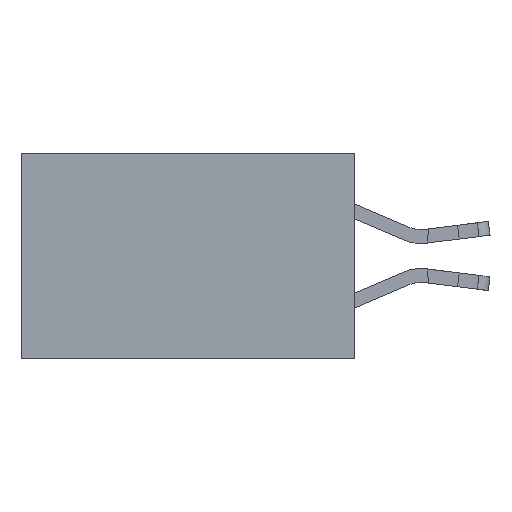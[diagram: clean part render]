
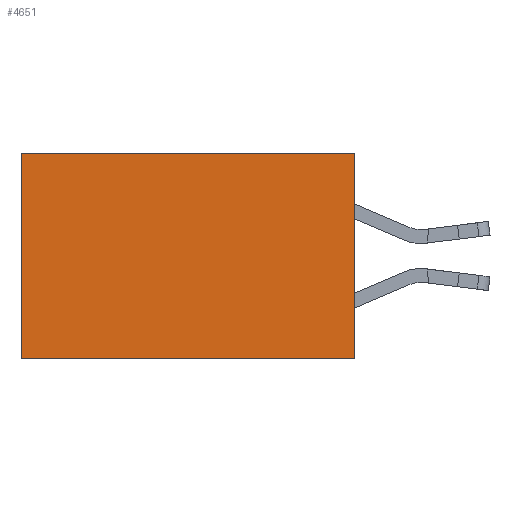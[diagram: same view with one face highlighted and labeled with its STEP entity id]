
A CAD part, left-side view. The second image highlights one B-rep face of the part: STEP entity #4651.
In plain terms, the highlighted planar face has unit normal (-1, 0, 0).
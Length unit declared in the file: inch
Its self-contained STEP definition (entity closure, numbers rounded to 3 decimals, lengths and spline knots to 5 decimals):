
#107 = CARTESIAN_POINT ( 'NONE',  ( 0.2615, 0.6, -0.37 ) ) ;
#495 = AXIS2_PLACEMENT_3D ( 'NONE', #16138, #16230, #9547 ) ;
#977 = VECTOR ( 'NONE', #4825, 39.37008 ) ;
#1746 = DIRECTION ( 'NONE',  ( 0., 1., 0. ) ) ;
#3487 = EDGE_CURVE ( 'NONE', #14373, #7581, #16564, .T. ) ;
#3870 = VECTOR ( 'NONE', #1746, 39.37008 ) ;
#4035 = EDGE_LOOP ( 'NONE', ( #16131, #14658, #6083, #10018 ) ) ;
#4062 = DIRECTION ( 'NONE',  ( 0., 0., -1. ) ) ;
#4365 = VERTEX_POINT ( 'NONE', #107 ) ;
#4651 = ADVANCED_FACE ( 'NONE', ( #12089 ), #7894, .F. ) ;
#4653 = CARTESIAN_POINT ( 'NONE',  ( 0.2615, 0.6, 0. ) ) ;
#4825 = DIRECTION ( 'NONE',  ( 0., 1., 0. ) ) ;
#5568 = CARTESIAN_POINT ( 'NONE',  ( 0.2615, 0., -0.37 ) ) ;
#6083 = ORIENTED_EDGE ( 'NONE', *, *, #12472, .F. ) ;
#6789 = LINE ( 'NONE', #5568, #12208 ) ;
#7273 = CARTESIAN_POINT ( 'NONE',  ( 0.2615, 0., -0.37 ) ) ;
#7565 = DIRECTION ( 'NONE',  ( 0., 0., -1. ) ) ;
#7581 = VERTEX_POINT ( 'NONE', #4653 ) ;
#7894 = PLANE ( 'NONE',  #495 ) ;
#9137 = EDGE_CURVE ( 'NONE', #7581, #4365, #15540, .T. ) ;
#9253 = VECTOR ( 'NONE', #7565, 39.37008 ) ;
#9547 = DIRECTION ( 'NONE',  ( 0., 0., -1. ) ) ;
#9799 = LINE ( 'NONE', #7273, #977 ) ;
#10018 = ORIENTED_EDGE ( 'NONE', *, *, #3487, .T. ) ;
#11276 = CARTESIAN_POINT ( 'NONE',  ( 0.2615, 0., -0.37 ) ) ;
#12089 = FACE_OUTER_BOUND ( 'NONE', #4035, .T. ) ;
#12208 = VECTOR ( 'NONE', #4062, 39.37008 ) ;
#12472 = EDGE_CURVE ( 'NONE', #14373, #15112, #6789, .T. ) ;
#12887 = CARTESIAN_POINT ( 'NONE',  ( 0.2615, 0., 0. ) ) ;
#14373 = VERTEX_POINT ( 'NONE', #12887 ) ;
#14658 = ORIENTED_EDGE ( 'NONE', *, *, #17177, .F. ) ;
#15085 = CARTESIAN_POINT ( 'NONE',  ( 0.2615, 0., 0. ) ) ;
#15112 = VERTEX_POINT ( 'NONE', #11276 ) ;
#15285 = CARTESIAN_POINT ( 'NONE',  ( 0.2615, 0.6, -0.37 ) ) ;
#15540 = LINE ( 'NONE', #15285, #9253 ) ;
#16131 = ORIENTED_EDGE ( 'NONE', *, *, #9137, .T. ) ;
#16138 = CARTESIAN_POINT ( 'NONE',  ( 0.2615, 0., -0.37 ) ) ;
#16230 = DIRECTION ( 'NONE',  ( 1., 0., 0. ) ) ;
#16564 = LINE ( 'NONE', #15085, #3870 ) ;
#17177 = EDGE_CURVE ( 'NONE', #15112, #4365, #9799, .T. ) ;
